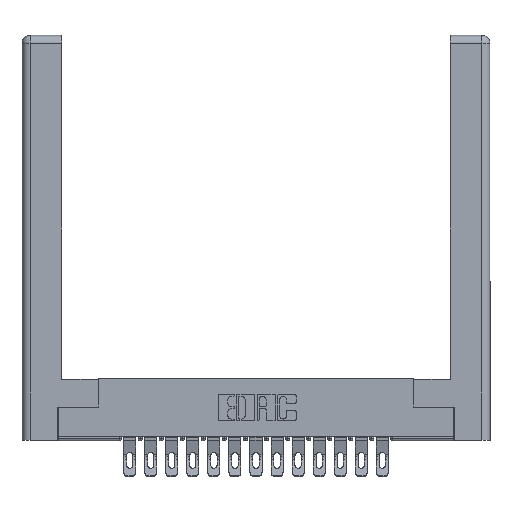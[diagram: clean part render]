
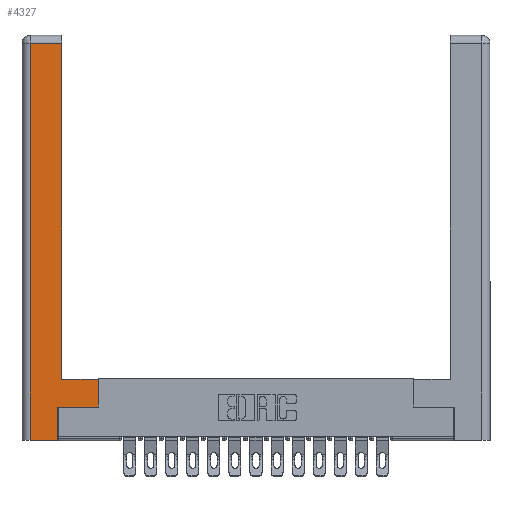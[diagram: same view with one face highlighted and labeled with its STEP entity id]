
A CAD part, top view. The second image highlights one B-rep face of the part: STEP entity #4327.
In plain terms, the highlighted planar face has unit normal (0, 0, 1).
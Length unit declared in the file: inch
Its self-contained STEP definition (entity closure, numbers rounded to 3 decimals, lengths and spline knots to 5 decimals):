
#78 = LINE ( 'NONE', #11456, #16725 ) ;
#346 = EDGE_CURVE ( 'NONE', #6876, #17636, #6995, .T. ) ;
#478 = VECTOR ( 'NONE', #19551, 39.37008 ) ;
#1011 = EDGE_CURVE ( 'NONE', #10768, #13531, #6207, .T. ) ;
#1126 = CARTESIAN_POINT ( 'NONE',  ( 0.295, 3., 0. ) ) ;
#2368 = ORIENTED_EDGE ( 'NONE', *, *, #11017, .T. ) ;
#3413 = CARTESIAN_POINT ( 'NONE',  ( 0.265, 0.245, 0. ) ) ;
#3965 = CARTESIAN_POINT ( 'NONE',  ( 0.295, 0.45, 0. ) ) ;
#4327 = ADVANCED_FACE ( 'NONE', ( #12563 ), #18874, .F. ) ;
#4339 = VERTEX_POINT ( 'NONE', #19646 ) ;
#4373 = DIRECTION ( 'NONE',  ( 0., 1., 0. ) ) ;
#4481 = LINE ( 'NONE', #3965, #18866 ) ;
#4816 = LINE ( 'NONE', #1126, #13162 ) ;
#5324 = DIRECTION ( 'NONE',  ( 0., 1., 0. ) ) ;
#5582 = ORIENTED_EDGE ( 'NONE', *, *, #10645, .T. ) ;
#5645 = ORIENTED_EDGE ( 'NONE', *, *, #7697, .T. ) ;
#5971 = VECTOR ( 'NONE', #5324, 39.37008 ) ;
#5981 = AXIS2_PLACEMENT_3D ( 'NONE', #11099, #9554, #20842 ) ;
#6207 = LINE ( 'NONE', #14742, #15309 ) ;
#6738 = DIRECTION ( 'NONE',  ( 0., -1., 0. ) ) ;
#6797 = CARTESIAN_POINT ( 'NONE',  ( 0.295, 2.94, 0. ) ) ;
#6876 = VERTEX_POINT ( 'NONE', #3413 ) ;
#6995 = LINE ( 'NONE', #8169, #478 ) ;
#7235 = LINE ( 'NONE', #13439, #18393 ) ;
#7263 = DIRECTION ( 'NONE',  ( -1., 0., 0. ) ) ;
#7429 = CARTESIAN_POINT ( 'NONE',  ( 0.0615, 2.94, 0. ) ) ;
#7697 = EDGE_CURVE ( 'NONE', #13531, #15839, #78, .T. ) ;
#7978 = LINE ( 'NONE', #13204, #10035 ) ;
#8169 = CARTESIAN_POINT ( 'NONE',  ( 0.565, 0.245, 0. ) ) ;
#8490 = EDGE_CURVE ( 'NONE', #18249, #18574, #4816, .T. ) ;
#9554 = DIRECTION ( 'NONE',  ( 0., 0., -1. ) ) ;
#10035 = VECTOR ( 'NONE', #11642, 39.37008 ) ;
#10270 = CARTESIAN_POINT ( 'NONE',  ( 0.565, 0.45, 0. ) ) ;
#10645 = EDGE_CURVE ( 'NONE', #18574, #10768, #7235, .T. ) ;
#10768 = VERTEX_POINT ( 'NONE', #7429 ) ;
#11017 = EDGE_CURVE ( 'NONE', #4339, #18249, #4481, .T. ) ;
#11099 = CARTESIAN_POINT ( 'NONE',  ( 0., 0., 0. ) ) ;
#11197 = EDGE_CURVE ( 'NONE', #17636, #4339, #11292, .T. ) ;
#11292 = LINE ( 'NONE', #10270, #5971 ) ;
#11456 = CARTESIAN_POINT ( 'NONE',  ( 0.265, 0., 0. ) ) ;
#11501 = EDGE_CURVE ( 'NONE', #15839, #6876, #7978, .T. ) ;
#11596 = EDGE_LOOP ( 'NONE', ( #11930, #5582, #19777, #5645, #12037, #15862, #20286, #2368 ) ) ;
#11642 = DIRECTION ( 'NONE',  ( 0., 1., 0. ) ) ;
#11930 = ORIENTED_EDGE ( 'NONE', *, *, #8490, .T. ) ;
#12037 = ORIENTED_EDGE ( 'NONE', *, *, #11501, .T. ) ;
#12563 = FACE_OUTER_BOUND ( 'NONE', #11596, .T. ) ;
#13143 = CARTESIAN_POINT ( 'NONE',  ( 0.295, 0.45, 0. ) ) ;
#13162 = VECTOR ( 'NONE', #4373, 39.37008 ) ;
#13204 = CARTESIAN_POINT ( 'NONE',  ( 0.265, 0.245, 0. ) ) ;
#13239 = DIRECTION ( 'NONE',  ( 1., 0., 0. ) ) ;
#13439 = CARTESIAN_POINT ( 'NONE',  ( 0.0615, 2.94, 0. ) ) ;
#13531 = VERTEX_POINT ( 'NONE', #19946 ) ;
#14742 = CARTESIAN_POINT ( 'NONE',  ( 0.0615, 0., 0. ) ) ;
#14839 = DIRECTION ( 'NONE',  ( -1., 0., 0. ) ) ;
#15309 = VECTOR ( 'NONE', #6738, 39.37008 ) ;
#15839 = VERTEX_POINT ( 'NONE', #19780 ) ;
#15862 = ORIENTED_EDGE ( 'NONE', *, *, #346, .T. ) ;
#16725 = VECTOR ( 'NONE', #13239, 39.37008 ) ;
#17636 = VERTEX_POINT ( 'NONE', #17827 ) ;
#17827 = CARTESIAN_POINT ( 'NONE',  ( 0.565, 0.245, 0. ) ) ;
#18249 = VERTEX_POINT ( 'NONE', #13143 ) ;
#18393 = VECTOR ( 'NONE', #14839, 39.37008 ) ;
#18574 = VERTEX_POINT ( 'NONE', #6797 ) ;
#18866 = VECTOR ( 'NONE', #7263, 39.37008 ) ;
#18874 = PLANE ( 'NONE',  #5981 ) ;
#19551 = DIRECTION ( 'NONE',  ( 1., 0., 0. ) ) ;
#19646 = CARTESIAN_POINT ( 'NONE',  ( 0.565, 0.45, 0. ) ) ;
#19777 = ORIENTED_EDGE ( 'NONE', *, *, #1011, .T. ) ;
#19780 = CARTESIAN_POINT ( 'NONE',  ( 0.265, 0., 0. ) ) ;
#19946 = CARTESIAN_POINT ( 'NONE',  ( 0.0615, 0., 0. ) ) ;
#20286 = ORIENTED_EDGE ( 'NONE', *, *, #11197, .T. ) ;
#20842 = DIRECTION ( 'NONE',  ( -1., 0., 0. ) ) ;
